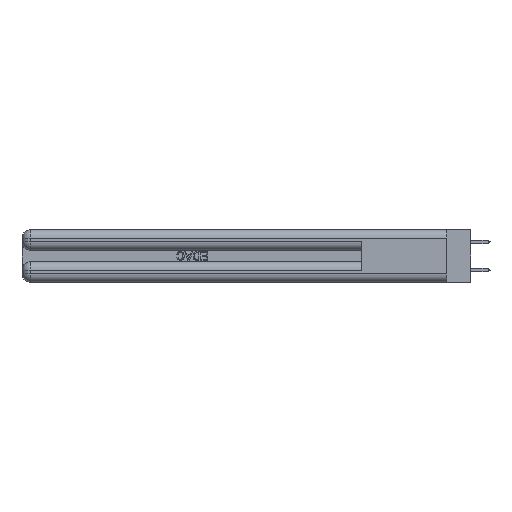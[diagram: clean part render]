
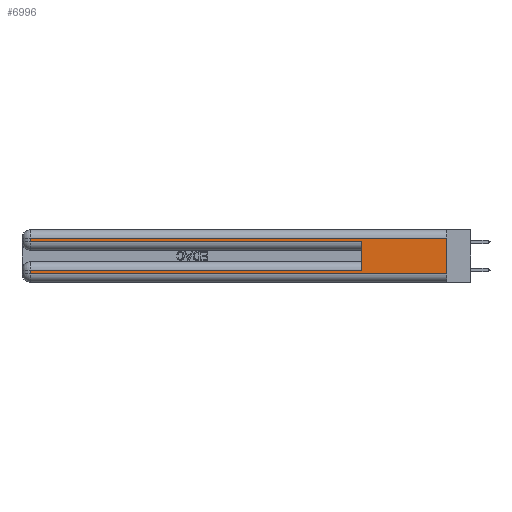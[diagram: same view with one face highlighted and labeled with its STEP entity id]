
A CAD part, left-side view. The second image highlights one B-rep face of the part: STEP entity #6996.
In plain terms, the highlighted planar face has unit normal (-1, 0, 0).
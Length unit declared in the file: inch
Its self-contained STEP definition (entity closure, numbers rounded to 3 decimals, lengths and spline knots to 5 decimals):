
#406 = VERTEX_POINT ( 'NONE', #17339 ) ;
#472 = EDGE_LOOP ( 'NONE', ( #30328, #5945, #33568, #5172, #31489, #17562, #24173, #31222 ) ) ;
#1135 = CARTESIAN_POINT ( 'NONE',  ( 0., 0.6, 0.285 ) ) ;
#2015 = LINE ( 'NONE', #9206, #17252 ) ;
#2144 = CARTESIAN_POINT ( 'NONE',  ( 0., 2.94, 0.06 ) ) ;
#2558 = CARTESIAN_POINT ( 'NONE',  ( 0., 2.94, 0.085 ) ) ;
#3187 = DIRECTION ( 'NONE',  ( 0., 0., 1. ) ) ;
#3739 = VERTEX_POINT ( 'NONE', #1135 ) ;
#4758 = CARTESIAN_POINT ( 'NONE',  ( 0., 0., 0.06 ) ) ;
#5172 = ORIENTED_EDGE ( 'NONE', *, *, #23778, .T. ) ;
#5945 = ORIENTED_EDGE ( 'NONE', *, *, #8423, .T. ) ;
#6425 = LINE ( 'NONE', #27208, #7379 ) ;
#6896 = DIRECTION ( 'NONE',  ( 0., 1., 0. ) ) ;
#6906 = CARTESIAN_POINT ( 'NONE',  ( 0., 2.94, 0.37 ) ) ;
#6996 = ADVANCED_FACE ( 'NONE', ( #28418 ), #8139, .F. ) ;
#7109 = EDGE_CURVE ( 'NONE', #29653, #22439, #6425, .T. ) ;
#7379 = VECTOR ( 'NONE', #27336, 39.37008 ) ;
#7648 = DIRECTION ( 'NONE',  ( 0., -1., 0. ) ) ;
#8139 = PLANE ( 'NONE',  #33053 ) ;
#8423 = EDGE_CURVE ( 'NONE', #29653, #21732, #12944, .T. ) ;
#8447 = VECTOR ( 'NONE', #26685, 39.37008 ) ;
#9206 = CARTESIAN_POINT ( 'NONE',  ( 0., 0.6, 0.145 ) ) ;
#10331 = VECTOR ( 'NONE', #6896, 39.37008 ) ;
#11784 = EDGE_CURVE ( 'NONE', #406, #25641, #20396, .T. ) ;
#12231 = LINE ( 'NONE', #36358, #8447 ) ;
#12887 = EDGE_CURVE ( 'NONE', #21732, #14393, #28084, .T. ) ;
#12944 = LINE ( 'NONE', #20408, #32155 ) ;
#13655 = VECTOR ( 'NONE', #31868, 39.37008 ) ;
#14393 = VERTEX_POINT ( 'NONE', #31556 ) ;
#14538 = DIRECTION ( 'NONE',  ( 0., 1., 0. ) ) ;
#16239 = VERTEX_POINT ( 'NONE', #2144 ) ;
#17252 = VECTOR ( 'NONE', #3187, 39.37008 ) ;
#17339 = CARTESIAN_POINT ( 'NONE',  ( 0., 0.6, 0.085 ) ) ;
#17562 = ORIENTED_EDGE ( 'NONE', *, *, #11784, .T. ) ;
#20020 = CARTESIAN_POINT ( 'NONE',  ( 0., 0., 0.37 ) ) ;
#20396 = LINE ( 'NONE', #24830, #10331 ) ;
#20408 = CARTESIAN_POINT ( 'NONE',  ( 0., 0., 0.31 ) ) ;
#20415 = DIRECTION ( 'NONE',  ( 0., 0., -1. ) ) ;
#21732 = VERTEX_POINT ( 'NONE', #35179 ) ;
#21765 = LINE ( 'NONE', #4758, #35212 ) ;
#22439 = VERTEX_POINT ( 'NONE', #26179 ) ;
#23778 = EDGE_CURVE ( 'NONE', #14393, #3739, #12231, .T. ) ;
#24173 = ORIENTED_EDGE ( 'NONE', *, *, #24196, .T. ) ;
#24196 = EDGE_CURVE ( 'NONE', #25641, #16239, #37154, .T. ) ;
#24279 = EDGE_CURVE ( 'NONE', #16239, #22439, #21765, .T. ) ;
#24830 = CARTESIAN_POINT ( 'NONE',  ( 0., 0., 0.085 ) ) ;
#25641 = VERTEX_POINT ( 'NONE', #2558 ) ;
#26179 = CARTESIAN_POINT ( 'NONE',  ( 0., 0., 0.06 ) ) ;
#26455 = CARTESIAN_POINT ( 'NONE',  ( 0., 0., 0.31 ) ) ;
#26685 = DIRECTION ( 'NONE',  ( 0., -1., 0. ) ) ;
#27160 = VECTOR ( 'NONE', #31363, 39.37008 ) ;
#27208 = CARTESIAN_POINT ( 'NONE',  ( 0., 0., 0.37 ) ) ;
#27336 = DIRECTION ( 'NONE',  ( 0., 0., -1. ) ) ;
#28084 = LINE ( 'NONE', #6906, #27160 ) ;
#28418 = FACE_OUTER_BOUND ( 'NONE', #472, .T. ) ;
#28499 = CARTESIAN_POINT ( 'NONE',  ( 0., 2.94, 0.37 ) ) ;
#29653 = VERTEX_POINT ( 'NONE', #26455 ) ;
#30328 = ORIENTED_EDGE ( 'NONE', *, *, #7109, .F. ) ;
#31222 = ORIENTED_EDGE ( 'NONE', *, *, #24279, .T. ) ;
#31363 = DIRECTION ( 'NONE',  ( 0., 0., -1. ) ) ;
#31489 = ORIENTED_EDGE ( 'NONE', *, *, #39386, .F. ) ;
#31556 = CARTESIAN_POINT ( 'NONE',  ( 0., 2.94, 0.285 ) ) ;
#31868 = DIRECTION ( 'NONE',  ( 0., 0., -1. ) ) ;
#32155 = VECTOR ( 'NONE', #14538, 39.37008 ) ;
#33053 = AXIS2_PLACEMENT_3D ( 'NONE', #20020, #38834, #20415 ) ;
#33568 = ORIENTED_EDGE ( 'NONE', *, *, #12887, .T. ) ;
#35179 = CARTESIAN_POINT ( 'NONE',  ( 0., 2.94, 0.31 ) ) ;
#35212 = VECTOR ( 'NONE', #7648, 39.37008 ) ;
#36358 = CARTESIAN_POINT ( 'NONE',  ( 0., 0., 0.285 ) ) ;
#37154 = LINE ( 'NONE', #28499, #13655 ) ;
#38834 = DIRECTION ( 'NONE',  ( 1., 0., 0. ) ) ;
#39386 = EDGE_CURVE ( 'NONE', #406, #3739, #2015, .T. ) ;
